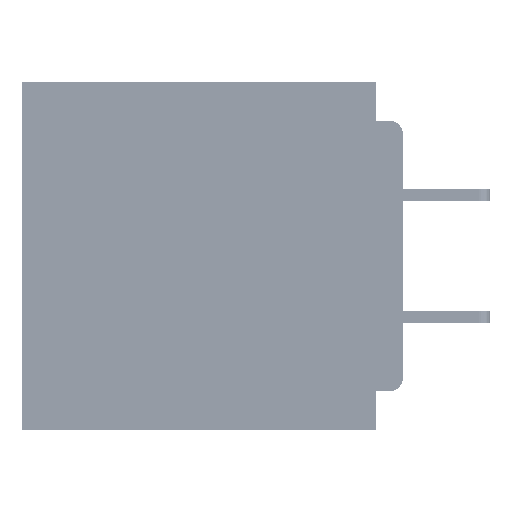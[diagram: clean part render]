
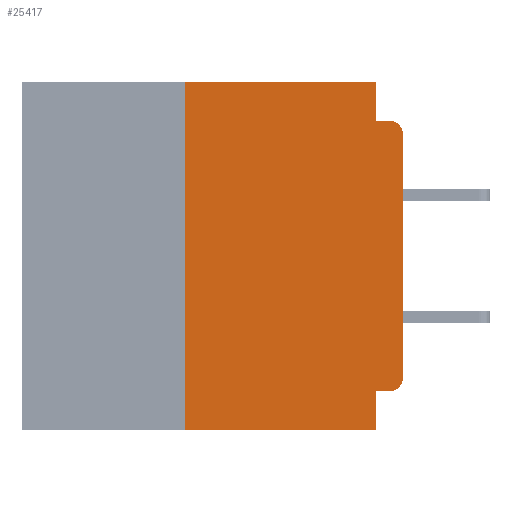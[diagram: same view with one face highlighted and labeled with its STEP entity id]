
A CAD part, left-side view. The second image highlights one B-rep face of the part: STEP entity #25417.
In plain terms, the highlighted planar face has unit normal (-1, 0, 0).
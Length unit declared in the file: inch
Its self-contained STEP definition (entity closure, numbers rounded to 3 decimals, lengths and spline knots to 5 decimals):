
#2072 = AXIS2_PLACEMENT_3D ( 'NONE', #12238, #50821, #17851 ) ;
#3229 = VECTOR ( 'NONE', #45481, 39.37008 ) ;
#3786 = VECTOR ( 'NONE', #52137, 39.37008 ) ;
#3844 = CARTESIAN_POINT ( 'NONE',  ( 0., 0.25, 0. ) ) ;
#4529 = AXIS2_PLACEMENT_3D ( 'NONE', #58955, #25960, #64470 ) ;
#4558 = CARTESIAN_POINT ( 'NONE',  ( 0., 0.031, 0. ) ) ;
#4934 = ORIENTED_EDGE ( 'NONE', *, *, #46596, .F. ) ;
#5187 = EDGE_LOOP ( 'NONE', ( #12235, #49785, #4934, #5729, #52585, #39481, #34184, #5958, #63128, #7421 ) ) ;
#5729 = ORIENTED_EDGE ( 'NONE', *, *, #51599, .F. ) ;
#5958 = ORIENTED_EDGE ( 'NONE', *, *, #13465, .F. ) ;
#6067 = VERTEX_POINT ( 'NONE', #3844 ) ;
#6700 = LINE ( 'NONE', #62107, #3229 ) ;
#7421 = ORIENTED_EDGE ( 'NONE', *, *, #44816, .T. ) ;
#8663 = VECTOR ( 'NONE', #15019, 39.37008 ) ;
#8938 = CARTESIAN_POINT ( 'NONE',  ( 0., 0.031, -0.355 ) ) ;
#10696 = CARTESIAN_POINT ( 'NONE',  ( 0., 0.015, -0.045 ) ) ;
#10820 = CARTESIAN_POINT ( 'NONE',  ( 0., 0.031, 0. ) ) ;
#11814 = CARTESIAN_POINT ( 'NONE',  ( 0., 0., -0.34 ) ) ;
#12235 = ORIENTED_EDGE ( 'NONE', *, *, #25096, .T. ) ;
#12238 = CARTESIAN_POINT ( 'NONE',  ( 0., 0.015, -0.06 ) ) ;
#12704 = CARTESIAN_POINT ( 'NONE',  ( 0., 0.031, -0.4 ) ) ;
#13465 = EDGE_CURVE ( 'NONE', #65630, #50668, #46130, .T. ) ;
#14724 = FACE_OUTER_BOUND ( 'NONE', #5187, .T. ) ;
#15019 = DIRECTION ( 'NONE',  ( 0., -1., 0. ) ) ;
#15811 = AXIS2_PLACEMENT_3D ( 'NONE', #29266, #51402, #18431 ) ;
#16471 = CARTESIAN_POINT ( 'NONE',  ( 0., 0., -0.355 ) ) ;
#17670 = VERTEX_POINT ( 'NONE', #67212 ) ;
#17851 = DIRECTION ( 'NONE',  ( 0., 0., -1. ) ) ;
#18431 = DIRECTION ( 'NONE',  ( 0., 0., -1. ) ) ;
#19160 = LINE ( 'NONE', #24518, #46709 ) ;
#19428 = VERTEX_POINT ( 'NONE', #11814 ) ;
#21994 = DIRECTION ( 'NONE',  ( 0., 0., 1. ) ) ;
#22704 = CIRCLE ( 'NONE', #2072, 0.015 ) ;
#23633 = LINE ( 'NONE', #4558, #54665 ) ;
#24404 = VECTOR ( 'NONE', #64637, 39.37008 ) ;
#24518 = CARTESIAN_POINT ( 'NONE',  ( 0., 0., 0. ) ) ;
#25096 = EDGE_CURVE ( 'NONE', #19428, #47208, #19160, .T. ) ;
#25417 = ADVANCED_FACE ( 'NONE', ( #14724 ), #45850, .F. ) ;
#25960 = DIRECTION ( 'NONE',  ( -1., 0., 0. ) ) ;
#26112 = LINE ( 'NONE', #59137, #24404 ) ;
#29266 = CARTESIAN_POINT ( 'NONE',  ( 0., 0.437, 0. ) ) ;
#31320 = VECTOR ( 'NONE', #21994, 39.37008 ) ;
#33050 = LINE ( 'NONE', #49431, #31320 ) ;
#33138 = EDGE_CURVE ( 'NONE', #34482, #65630, #66804, .T. ) ;
#33140 = DIRECTION ( 'NONE',  ( 0., 1., 0. ) ) ;
#34184 = ORIENTED_EDGE ( 'NONE', *, *, #58054, .T. ) ;
#34482 = VERTEX_POINT ( 'NONE', #64380 ) ;
#35113 = CARTESIAN_POINT ( 'NONE',  ( 0., 0.031, -0.045 ) ) ;
#35589 = DIRECTION ( 'NONE',  ( 0., 0., 1. ) ) ;
#36579 = VERTEX_POINT ( 'NONE', #10820 ) ;
#37344 = EDGE_CURVE ( 'NONE', #6067, #36579, #26112, .T. ) ;
#39481 = ORIENTED_EDGE ( 'NONE', *, *, #68838, .F. ) ;
#43204 = DIRECTION ( 'NONE',  ( 0., 0., -1. ) ) ;
#44816 = EDGE_CURVE ( 'NONE', #34482, #19428, #47608, .T. ) ;
#45481 = DIRECTION ( 'NONE',  ( 0., -1., 0. ) ) ;
#45850 = PLANE ( 'NONE',  #15811 ) ;
#46130 = LINE ( 'NONE', #57693, #3786 ) ;
#46596 = EDGE_CURVE ( 'NONE', #59662, #47050, #6700, .T. ) ;
#46709 = VECTOR ( 'NONE', #35589, 39.37008 ) ;
#47050 = VERTEX_POINT ( 'NONE', #10696 ) ;
#47208 = VERTEX_POINT ( 'NONE', #56279 ) ;
#47608 = CIRCLE ( 'NONE', #4529, 0.015 ) ;
#48098 = CARTESIAN_POINT ( 'NONE',  ( 0., 0.437, -0.4 ) ) ;
#49431 = CARTESIAN_POINT ( 'NONE',  ( 0., 0.25, -0.4 ) ) ;
#49785 = ORIENTED_EDGE ( 'NONE', *, *, #69021, .T. ) ;
#50668 = VERTEX_POINT ( 'NONE', #12704 ) ;
#50821 = DIRECTION ( 'NONE',  ( -1., 0., 0. ) ) ;
#50950 = LINE ( 'NONE', #48098, #8663 ) ;
#51402 = DIRECTION ( 'NONE',  ( 1., 0., 0. ) ) ;
#51599 = EDGE_CURVE ( 'NONE', #36579, #59662, #23633, .T. ) ;
#52137 = DIRECTION ( 'NONE',  ( 0., 0., -1. ) ) ;
#52177 = VECTOR ( 'NONE', #33140, 39.37008 ) ;
#52585 = ORIENTED_EDGE ( 'NONE', *, *, #37344, .F. ) ;
#54665 = VECTOR ( 'NONE', #43204, 39.37008 ) ;
#56279 = CARTESIAN_POINT ( 'NONE',  ( 0., 0., -0.06 ) ) ;
#57693 = CARTESIAN_POINT ( 'NONE',  ( 0., 0.031, -0.4 ) ) ;
#58054 = EDGE_CURVE ( 'NONE', #17670, #50668, #50950, .T. ) ;
#58955 = CARTESIAN_POINT ( 'NONE',  ( 0., 0.015, -0.34 ) ) ;
#59137 = CARTESIAN_POINT ( 'NONE',  ( 0., 0.437, 0. ) ) ;
#59662 = VERTEX_POINT ( 'NONE', #35113 ) ;
#62107 = CARTESIAN_POINT ( 'NONE',  ( 0., 0., -0.045 ) ) ;
#63128 = ORIENTED_EDGE ( 'NONE', *, *, #33138, .F. ) ;
#64380 = CARTESIAN_POINT ( 'NONE',  ( 0., 0.015, -0.355 ) ) ;
#64470 = DIRECTION ( 'NONE',  ( 0., 0., -1. ) ) ;
#64637 = DIRECTION ( 'NONE',  ( 0., -1., 0. ) ) ;
#65630 = VERTEX_POINT ( 'NONE', #8938 ) ;
#66804 = LINE ( 'NONE', #16471, #52177 ) ;
#67212 = CARTESIAN_POINT ( 'NONE',  ( 0., 0.25, -0.4 ) ) ;
#68838 = EDGE_CURVE ( 'NONE', #17670, #6067, #33050, .T. ) ;
#69021 = EDGE_CURVE ( 'NONE', #47208, #47050, #22704, .T. ) ;
